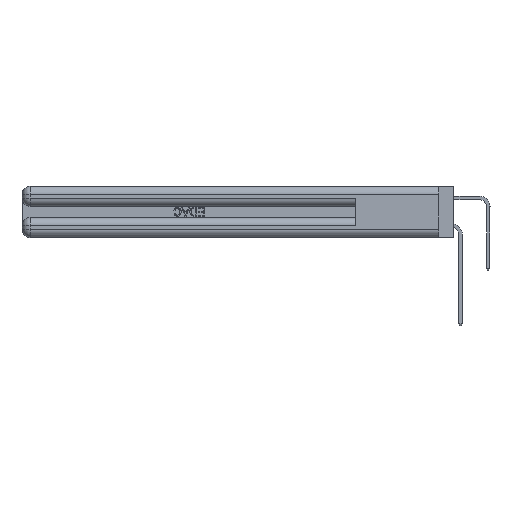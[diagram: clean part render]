
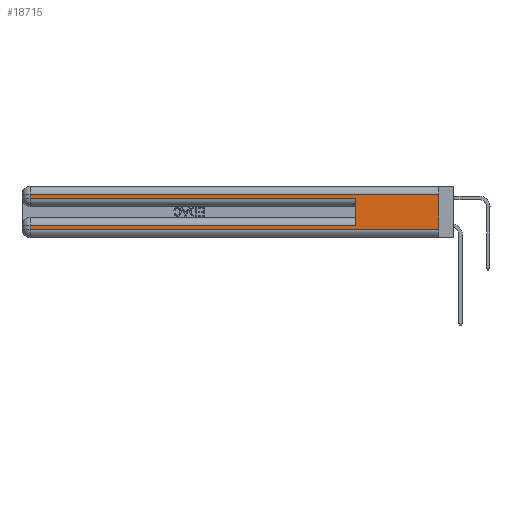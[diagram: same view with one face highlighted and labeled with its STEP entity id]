
A CAD part, left-side view. The second image highlights one B-rep face of the part: STEP entity #18715.
In plain terms, the highlighted planar face has unit normal (-1, 0, 0).
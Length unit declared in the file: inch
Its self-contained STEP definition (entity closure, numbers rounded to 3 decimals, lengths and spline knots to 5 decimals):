
#19 = PLANE ( 'NONE',  #13851 ) ;
#1263 = CARTESIAN_POINT ( 'NONE',  ( 0., 2.94, 0.37 ) ) ;
#1990 = CARTESIAN_POINT ( 'NONE',  ( 0., 2.94, 0.31 ) ) ;
#2854 = ORIENTED_EDGE ( 'NONE', *, *, #14682, .F. ) ;
#3318 = LINE ( 'NONE', #19404, #42444 ) ;
#3876 = DIRECTION ( 'NONE',  ( 1., 0., 0. ) ) ;
#5054 = LINE ( 'NONE', #28490, #14018 ) ;
#5594 = CARTESIAN_POINT ( 'NONE',  ( 0., 2.94, 0.285 ) ) ;
#5775 = EDGE_CURVE ( 'NONE', #14429, #12841, #17791, .T. ) ;
#6136 = EDGE_CURVE ( 'NONE', #47148, #34583, #41401, .T. ) ;
#9419 = ORIENTED_EDGE ( 'NONE', *, *, #30338, .T. ) ;
#10977 = DIRECTION ( 'NONE',  ( 0., -1., 0. ) ) ;
#11791 = CARTESIAN_POINT ( 'NONE',  ( 0., 0., 0.37 ) ) ;
#12841 = VERTEX_POINT ( 'NONE', #30920 ) ;
#13851 = AXIS2_PLACEMENT_3D ( 'NONE', #34135, #3876, #30511 ) ;
#14018 = VECTOR ( 'NONE', #32253, 39.37008 ) ;
#14415 = DIRECTION ( 'NONE',  ( 0., 0., -1. ) ) ;
#14429 = VERTEX_POINT ( 'NONE', #43403 ) ;
#14682 = EDGE_CURVE ( 'NONE', #14429, #26331, #17144, .T. ) ;
#16981 = CARTESIAN_POINT ( 'NONE',  ( 0., 0.6, 0.145 ) ) ;
#17057 = VERTEX_POINT ( 'NONE', #45465 ) ;
#17144 = LINE ( 'NONE', #16981, #36141 ) ;
#17755 = FACE_OUTER_BOUND ( 'NONE', #46718, .T. ) ;
#17791 = LINE ( 'NONE', #31604, #26762 ) ;
#18715 = ADVANCED_FACE ( 'NONE', ( #17755 ), #19, .F. ) ;
#19404 = CARTESIAN_POINT ( 'NONE',  ( 0., 0., 0.31 ) ) ;
#20856 = DIRECTION ( 'NONE',  ( 0., 0., 1. ) ) ;
#21589 = VECTOR ( 'NONE', #14415, 39.37008 ) ;
#23795 = ORIENTED_EDGE ( 'NONE', *, *, #6136, .T. ) ;
#26331 = VERTEX_POINT ( 'NONE', #36180 ) ;
#26349 = ORIENTED_EDGE ( 'NONE', *, *, #34458, .T. ) ;
#26762 = VECTOR ( 'NONE', #46678, 39.37008 ) ;
#28490 = CARTESIAN_POINT ( 'NONE',  ( 0., 0., 0.285 ) ) ;
#29568 = CARTESIAN_POINT ( 'NONE',  ( 0., 2.94, 0.37 ) ) ;
#29785 = CARTESIAN_POINT ( 'NONE',  ( 0., 0., 0.06 ) ) ;
#30227 = VECTOR ( 'NONE', #10977, 39.37008 ) ;
#30338 = EDGE_CURVE ( 'NONE', #41164, #46953, #34605, .T. ) ;
#30511 = DIRECTION ( 'NONE',  ( 0., 0., -1. ) ) ;
#30624 = EDGE_CURVE ( 'NONE', #12841, #47148, #31590, .T. ) ;
#30920 = CARTESIAN_POINT ( 'NONE',  ( 0., 2.94, 0.085 ) ) ;
#31471 = CARTESIAN_POINT ( 'NONE',  ( 0., 0., 0.06 ) ) ;
#31590 = LINE ( 'NONE', #29568, #21589 ) ;
#31604 = CARTESIAN_POINT ( 'NONE',  ( 0., 0., 0.085 ) ) ;
#32253 = DIRECTION ( 'NONE',  ( 0., -1., 0. ) ) ;
#32619 = ORIENTED_EDGE ( 'NONE', *, *, #30624, .T. ) ;
#33451 = ORIENTED_EDGE ( 'NONE', *, *, #48561, .F. ) ;
#34135 = CARTESIAN_POINT ( 'NONE',  ( 0., 0., 0.37 ) ) ;
#34458 = EDGE_CURVE ( 'NONE', #17057, #41164, #3318, .T. ) ;
#34583 = VERTEX_POINT ( 'NONE', #31471 ) ;
#34605 = LINE ( 'NONE', #1263, #43365 ) ;
#36141 = VECTOR ( 'NONE', #20856, 39.37008 ) ;
#36180 = CARTESIAN_POINT ( 'NONE',  ( 0., 0.6, 0.285 ) ) ;
#37315 = CARTESIAN_POINT ( 'NONE',  ( 0., 2.94, 0.06 ) ) ;
#38319 = DIRECTION ( 'NONE',  ( 0., 0., -1. ) ) ;
#39114 = DIRECTION ( 'NONE',  ( 0., 0., -1. ) ) ;
#39655 = ORIENTED_EDGE ( 'NONE', *, *, #46404, .T. ) ;
#39880 = LINE ( 'NONE', #11791, #41051 ) ;
#41051 = VECTOR ( 'NONE', #38319, 39.37008 ) ;
#41164 = VERTEX_POINT ( 'NONE', #1990 ) ;
#41401 = LINE ( 'NONE', #29785, #30227 ) ;
#42158 = DIRECTION ( 'NONE',  ( 0., 1., 0. ) ) ;
#42444 = VECTOR ( 'NONE', #42158, 39.37008 ) ;
#43365 = VECTOR ( 'NONE', #39114, 39.37008 ) ;
#43403 = CARTESIAN_POINT ( 'NONE',  ( 0., 0.6, 0.085 ) ) ;
#45465 = CARTESIAN_POINT ( 'NONE',  ( 0., 0., 0.31 ) ) ;
#46404 = EDGE_CURVE ( 'NONE', #46953, #26331, #5054, .T. ) ;
#46678 = DIRECTION ( 'NONE',  ( 0., 1., 0. ) ) ;
#46718 = EDGE_LOOP ( 'NONE', ( #33451, #26349, #9419, #39655, #2854, #49012, #32619, #23795 ) ) ;
#46953 = VERTEX_POINT ( 'NONE', #5594 ) ;
#47148 = VERTEX_POINT ( 'NONE', #37315 ) ;
#48561 = EDGE_CURVE ( 'NONE', #17057, #34583, #39880, .T. ) ;
#49012 = ORIENTED_EDGE ( 'NONE', *, *, #5775, .T. ) ;
